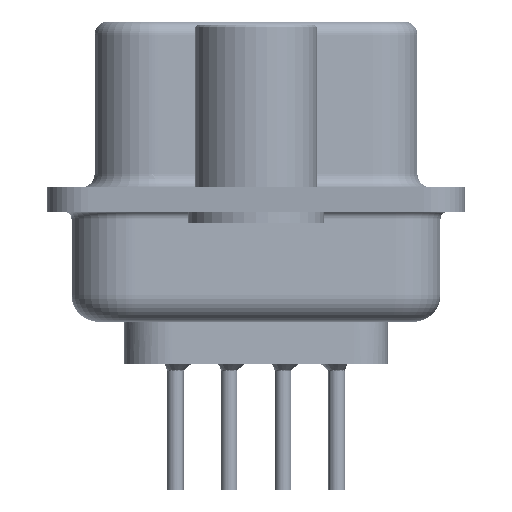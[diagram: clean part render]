
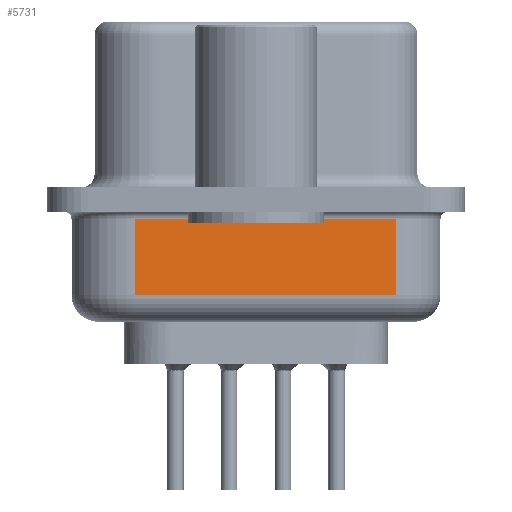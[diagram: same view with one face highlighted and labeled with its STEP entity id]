
A CAD part, left-side view. The second image highlights one B-rep face of the part: STEP entity #5731.
In plain terms, the highlighted planar face has unit normal (-0.985, -0.174, 0).
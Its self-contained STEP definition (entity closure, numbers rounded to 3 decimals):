
#755 = CARTESIAN_POINT ( 'NONE',  ( 4.723, -5.147, -3.5 ) ) ;
#767 = VERTEX_POINT ( 'NONE', #37556 ) ;
#824 = LINE ( 'NONE', #12136, #8576 ) ;
#1139 = CARTESIAN_POINT ( 'NONE',  ( 3.03, 4.453, -4.5 ) ) ;
#1354 = FACE_OUTER_BOUND ( 'NONE', #17862, .T. ) ;
#3111 = DIRECTION ( 'NONE',  ( -0.174, 0.985, 0. ) ) ;
#5717 = VECTOR ( 'NONE', #16043, 1000. ) ;
#5731 = ADVANCED_FACE ( 'NONE', ( #1354 ), #16032, .F. ) ;
#6520 = CARTESIAN_POINT ( 'NONE',  ( 4.723, -5.147, -0.7 ) ) ;
#6826 = ORIENTED_EDGE ( 'NONE', *, *, #40265, .F. ) ;
#7075 = VERTEX_POINT ( 'NONE', #6520 ) ;
#8576 = VECTOR ( 'NONE', #22963, 1000. ) ;
#12136 = CARTESIAN_POINT ( 'NONE',  ( 4.723, -5.147, -4.5 ) ) ;
#12431 = DIRECTION ( 'NONE',  ( 0.174, -0.985, 0. ) ) ;
#15573 = LINE ( 'NONE', #1139, #5717 ) ;
#16032 = PLANE ( 'NONE',  #39949 ) ;
#16043 = DIRECTION ( 'NONE',  ( 0., 0., 1. ) ) ;
#17862 = EDGE_LOOP ( 'NONE', ( #6826, #26386, #25010, #26149 ) ) ;
#22963 = DIRECTION ( 'NONE',  ( 0., 0., 1. ) ) ;
#25010 = ORIENTED_EDGE ( 'NONE', *, *, #44838, .T. ) ;
#26149 = ORIENTED_EDGE ( 'NONE', *, *, #35392, .T. ) ;
#26386 = ORIENTED_EDGE ( 'NONE', *, *, #38968, .T. ) ;
#27779 = DIRECTION ( 'NONE',  ( -0.174, 0.985, 0. ) ) ;
#32402 = CARTESIAN_POINT ( 'NONE',  ( 3.03, 4.453, -0.7 ) ) ;
#34935 = VECTOR ( 'NONE', #12431, 1000. ) ;
#35392 = EDGE_CURVE ( 'NONE', #7075, #35741, #46899, .T. ) ;
#35741 = VERTEX_POINT ( 'NONE', #32402 ) ;
#36077 = CARTESIAN_POINT ( 'NONE',  ( 3.03, 4.453, -0.7 ) ) ;
#36174 = VECTOR ( 'NONE', #3111, 1000. ) ;
#37212 = CARTESIAN_POINT ( 'NONE',  ( 3.03, 4.453, -3.5 ) ) ;
#37556 = CARTESIAN_POINT ( 'NONE',  ( 3.03, 4.453, -3.5 ) ) ;
#37672 = DIRECTION ( 'NONE',  ( 0.985, 0.174, 0. ) ) ;
#37846 = VERTEX_POINT ( 'NONE', #755 ) ;
#38968 = EDGE_CURVE ( 'NONE', #767, #37846, #41500, .T. ) ;
#39949 = AXIS2_PLACEMENT_3D ( 'NONE', #45343, #37672, #27779 ) ;
#40265 = EDGE_CURVE ( 'NONE', #767, #35741, #15573, .T. ) ;
#41500 = LINE ( 'NONE', #37212, #34935 ) ;
#44838 = EDGE_CURVE ( 'NONE', #37846, #7075, #824, .T. ) ;
#45343 = CARTESIAN_POINT ( 'NONE',  ( 3.03, 4.453, -4.5 ) ) ;
#46899 = LINE ( 'NONE', #36077, #36174 ) ;
